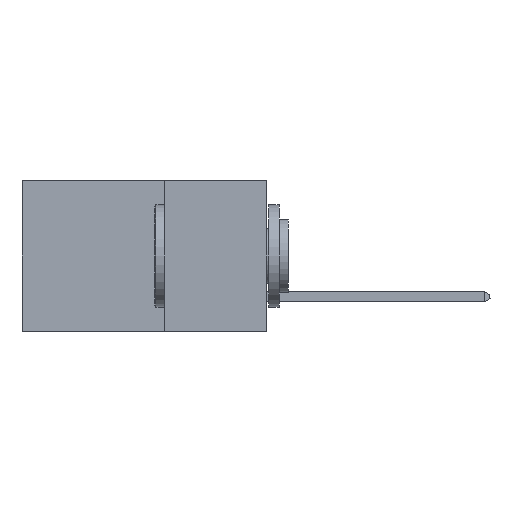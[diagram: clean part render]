
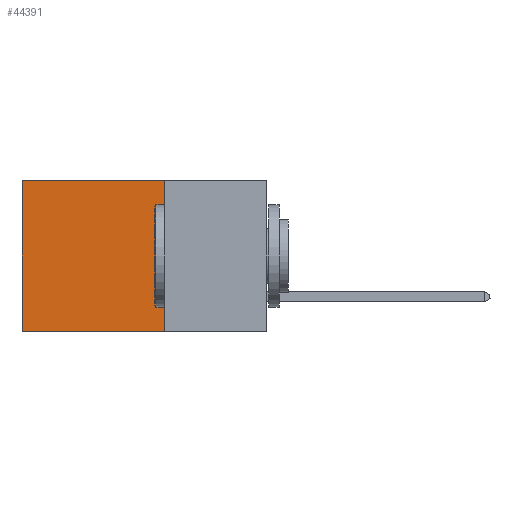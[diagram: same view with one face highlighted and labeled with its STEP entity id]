
A CAD part, left-side view. The second image highlights one B-rep face of the part: STEP entity #44391.
In plain terms, the highlighted planar face has unit normal (-1, 0, 0).
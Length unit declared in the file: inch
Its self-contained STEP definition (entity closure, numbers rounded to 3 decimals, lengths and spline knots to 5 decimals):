
#3144 = VERTEX_POINT ( 'NONE', #42144 ) ;
#3863 = CARTESIAN_POINT ( 'NONE',  ( 0.2875, 0.6, 0. ) ) ;
#4766 = VECTOR ( 'NONE', #16188, 39.37008 ) ;
#5338 = EDGE_CURVE ( 'NONE', #3144, #43080, #34712, .T. ) ;
#6121 = DIRECTION ( 'NONE',  ( 0., 1., 0. ) ) ;
#7767 = CARTESIAN_POINT ( 'NONE',  ( 0.2875, 0.25, 0. ) ) ;
#8625 = VERTEX_POINT ( 'NONE', #3863 ) ;
#11077 = EDGE_CURVE ( 'NONE', #8625, #43110, #23033, .T. ) ;
#11107 = CARTESIAN_POINT ( 'NONE',  ( 0.2875, 0.6, 0. ) ) ;
#13125 = CARTESIAN_POINT ( 'NONE',  ( 0.2875, 0.25, -0.37 ) ) ;
#14467 = EDGE_CURVE ( 'NONE', #43080, #43110, #28955, .T. ) ;
#15482 = DIRECTION ( 'NONE',  ( 0., 0., -1. ) ) ;
#15736 = CARTESIAN_POINT ( 'NONE',  ( 0.2875, 0.6, -0.37 ) ) ;
#16188 = DIRECTION ( 'NONE',  ( 0., 1., 0. ) ) ;
#21070 = CARTESIAN_POINT ( 'NONE',  ( 0.2875, 0.25, 0. ) ) ;
#21233 = VECTOR ( 'NONE', #15482, 39.37008 ) ;
#23033 = LINE ( 'NONE', #11107, #21233 ) ;
#24916 = ORIENTED_EDGE ( 'NONE', *, *, #11077, .T. ) ;
#26158 = EDGE_LOOP ( 'NONE', ( #24916, #39683, #30946, #48757 ) ) ;
#27475 = FACE_OUTER_BOUND ( 'NONE', #26158, .T. ) ;
#28717 = CARTESIAN_POINT ( 'NONE',  ( 0.2875, 0.25, -0.37 ) ) ;
#28955 = LINE ( 'NONE', #28717, #35387 ) ;
#30785 = DIRECTION ( 'NONE',  ( 1., 0., 0. ) ) ;
#30938 = CARTESIAN_POINT ( 'NONE',  ( 0.2875, 0.25, 0. ) ) ;
#30946 = ORIENTED_EDGE ( 'NONE', *, *, #5338, .F. ) ;
#31990 = LINE ( 'NONE', #7767, #4766 ) ;
#32036 = EDGE_CURVE ( 'NONE', #3144, #8625, #31990, .T. ) ;
#34649 = AXIS2_PLACEMENT_3D ( 'NONE', #30938, #30785, #38858 ) ;
#34712 = LINE ( 'NONE', #21070, #41839 ) ;
#34887 = PLANE ( 'NONE',  #34649 ) ;
#35387 = VECTOR ( 'NONE', #6121, 39.37008 ) ;
#36361 = DIRECTION ( 'NONE',  ( 0., 0., -1. ) ) ;
#38858 = DIRECTION ( 'NONE',  ( 0., 0., -1. ) ) ;
#39683 = ORIENTED_EDGE ( 'NONE', *, *, #14467, .F. ) ;
#41839 = VECTOR ( 'NONE', #36361, 39.37008 ) ;
#42144 = CARTESIAN_POINT ( 'NONE',  ( 0.2875, 0.25, 0. ) ) ;
#43080 = VERTEX_POINT ( 'NONE', #13125 ) ;
#43110 = VERTEX_POINT ( 'NONE', #15736 ) ;
#44391 = ADVANCED_FACE ( 'NONE', ( #27475 ), #34887, .F. ) ;
#48757 = ORIENTED_EDGE ( 'NONE', *, *, #32036, .T. ) ;
